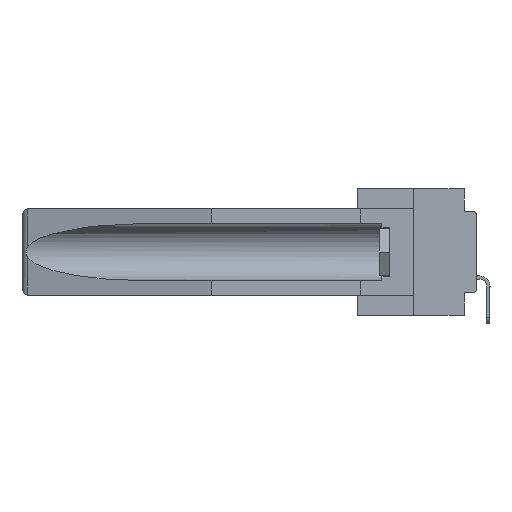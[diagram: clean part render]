
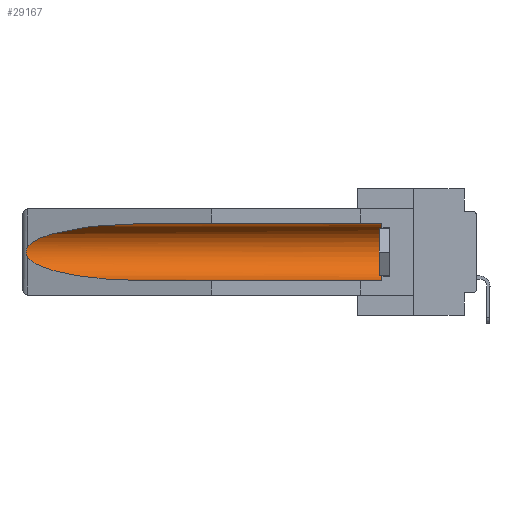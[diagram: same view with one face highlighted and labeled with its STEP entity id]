
A CAD part, left-side view. The second image highlights one B-rep face of the part: STEP entity #29167.
In plain terms, the highlighted cylindrical face has radius 2.857 mm (diameter 5.715 mm), a partial arc.
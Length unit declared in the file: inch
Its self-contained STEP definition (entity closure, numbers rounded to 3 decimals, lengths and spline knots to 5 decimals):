
#1202 = CARTESIAN_POINT ( 'NONE',  ( 0.26597, 1.5296, -0.19026 ) ) ;
#1560 = CARTESIAN_POINT ( 'NONE',  ( 0.21114, 1.30732, -0.284 ) ) ;
#1847 = AXIS2_PLACEMENT_3D ( 'NONE', #2452, #24636, #7703 ) ;
#2257 =( BOUNDED_CURVE ( )  B_SPLINE_CURVE ( 3, ( #26193, #17725, #25839, #3840 ),
 .UNSPECIFIED., .F., .F. ) 
 B_SPLINE_CURVE_WITH_KNOTS ( ( 4, 4 ),
 ( 4.71239, 6.08839 ),
 .UNSPECIFIED. ) 
 CURVE ( )  GEOMETRIC_REPRESENTATION_ITEM ( )  RATIONAL_B_SPLINE_CURVE ( ( 1., 0.848, 0.848, 1. ) ) 
 REPRESENTATION_ITEM ( '' )  );
#2452 = CARTESIAN_POINT ( 'NONE',  ( 0.155, -0.30754, -0.1715 ) ) ;
#2666 = EDGE_CURVE ( 'NONE', #32595, #31983, #2257, .T. ) ;
#3594 = VERTEX_POINT ( 'NONE', #14603 ) ;
#3840 = CARTESIAN_POINT ( 'NONE',  ( 0.26537, 1.52718, -0.14972 ) ) ;
#4075 = CIRCLE ( 'NONE', #16179, 0.1125 ) ;
#4083 = CARTESIAN_POINT ( 'NONE',  ( 0.26655, 1.53094, -0.18657 ) ) ;
#4867 = LINE ( 'NONE', #29758, #33152 ) ;
#6982 = EDGE_LOOP ( 'NONE', ( #12656, #14835, #35132, #25959, #32032, #20372 ) ) ;
#7193 = LINE ( 'NONE', #20549, #9250 ) ;
#7543 =( BOUNDED_CURVE ( )  B_SPLINE_CURVE ( 3, ( #23751, #20517, #1560, #31512 ),
 .UNSPECIFIED., .F., .F. ) 
 B_SPLINE_CURVE_WITH_KNOTS ( ( 4, 4 ),
 ( 0.1948, 1.5708 ),
 .UNSPECIFIED. ) 
 CURVE ( )  GEOMETRIC_REPRESENTATION_ITEM ( )  RATIONAL_B_SPLINE_CURVE ( ( 1., 0.848, 0.848, 1. ) ) 
 REPRESENTATION_ITEM ( '' )  );
#7703 = DIRECTION ( 'NONE',  ( 0., 0., 1. ) ) ;
#7984 = B_SPLINE_CURVE_WITH_KNOTS ( 'NONE', 3,
 ( #17441, #28968, #20332, #14750, #31323, #28789, #28255, #4083, #1202, #12393 ),
 .UNSPECIFIED., .F., .F.,
 ( 4, 2, 2, 2, 4 ),
 ( 0., 0.00029, 0.00058, 0.00087, 0.00117 ),
 .UNSPECIFIED. ) ;
#9250 = VECTOR ( 'NONE', #15162, 39.37008 ) ;
#10125 = CARTESIAN_POINT ( 'NONE',  ( 0.155, 0.126, -0.284 ) ) ;
#10772 = VERTEX_POINT ( 'NONE', #26915 ) ;
#11515 = EDGE_CURVE ( 'NONE', #10772, #3594, #7543, .T. ) ;
#12393 = CARTESIAN_POINT ( 'NONE',  ( 0.26537, 1.52718, -0.19328 ) ) ;
#12656 = ORIENTED_EDGE ( 'NONE', *, *, #2666, .T. ) ;
#14603 = CARTESIAN_POINT ( 'NONE',  ( 0.155, 1.07973, -0.284 ) ) ;
#14750 = CARTESIAN_POINT ( 'NONE',  ( 0.2673, 1.5327, -0.16383 ) ) ;
#14835 = ORIENTED_EDGE ( 'NONE', *, *, #24564, .T. ) ;
#15162 = DIRECTION ( 'NONE',  ( 0., 1., 0. ) ) ;
#16179 = AXIS2_PLACEMENT_3D ( 'NONE', #34949, #31898, #29348 ) ;
#16348 = EDGE_CURVE ( 'NONE', #18946, #3594, #4867, .T. ) ;
#16714 = FACE_OUTER_BOUND ( 'NONE', #6982, .T. ) ;
#17441 = CARTESIAN_POINT ( 'NONE',  ( 0.26537, 1.52718, -0.14972 ) ) ;
#17725 = CARTESIAN_POINT ( 'NONE',  ( 0.21114, 1.30732, -0.059 ) ) ;
#18946 = VERTEX_POINT ( 'NONE', #10125 ) ;
#20332 = CARTESIAN_POINT ( 'NONE',  ( 0.26654, 1.53092, -0.15636 ) ) ;
#20372 = ORIENTED_EDGE ( 'NONE', *, *, #20617, .T. ) ;
#20517 = CARTESIAN_POINT ( 'NONE',  ( 0.25451, 1.48313, -0.24835 ) ) ;
#20549 = CARTESIAN_POINT ( 'NONE',  ( 0.155, -0.30754, -0.059 ) ) ;
#20617 = EDGE_CURVE ( 'NONE', #28880, #32595, #7193, .T. ) ;
#22952 = EDGE_CURVE ( 'NONE', #18946, #28880, #4075, .T. ) ;
#23751 = CARTESIAN_POINT ( 'NONE',  ( 0.26537, 1.52718, -0.19328 ) ) ;
#24564 = EDGE_CURVE ( 'NONE', #31983, #10772, #7984, .T. ) ;
#24636 = DIRECTION ( 'NONE',  ( 0., 1., 0. ) ) ;
#24831 = CYLINDRICAL_SURFACE ( 'NONE', #1847, 0.1125 ) ;
#25839 = CARTESIAN_POINT ( 'NONE',  ( 0.25451, 1.48313, -0.09465 ) ) ;
#25959 = ORIENTED_EDGE ( 'NONE', *, *, #16348, .F. ) ;
#26193 = CARTESIAN_POINT ( 'NONE',  ( 0.155, 1.07973, -0.059 ) ) ;
#26869 = DIRECTION ( 'NONE',  ( 0., 1., 0. ) ) ;
#26915 = CARTESIAN_POINT ( 'NONE',  ( 0.26537, 1.52718, -0.19328 ) ) ;
#28255 = CARTESIAN_POINT ( 'NONE',  ( 0.2673, 1.53269, -0.17917 ) ) ;
#28539 = CARTESIAN_POINT ( 'NONE',  ( 0.155, 1.07973, -0.059 ) ) ;
#28627 = CARTESIAN_POINT ( 'NONE',  ( 0.155, 0.126, -0.059 ) ) ;
#28789 = CARTESIAN_POINT ( 'NONE',  ( 0.2675, 1.53308, -0.17534 ) ) ;
#28880 = VERTEX_POINT ( 'NONE', #28627 ) ;
#28968 = CARTESIAN_POINT ( 'NONE',  ( 0.26597, 1.52961, -0.15275 ) ) ;
#29167 = ADVANCED_FACE ( 'NONE', ( #16714 ), #24831, .F. ) ;
#29348 = DIRECTION ( 'NONE',  ( 0., 0., 1. ) ) ;
#29758 = CARTESIAN_POINT ( 'NONE',  ( 0.155, -0.30754, -0.284 ) ) ;
#31323 = CARTESIAN_POINT ( 'NONE',  ( 0.2675, 1.53308, -0.16763 ) ) ;
#31512 = CARTESIAN_POINT ( 'NONE',  ( 0.155, 1.07973, -0.284 ) ) ;
#31898 = DIRECTION ( 'NONE',  ( 0., -1., 0. ) ) ;
#31983 = VERTEX_POINT ( 'NONE', #33147 ) ;
#32032 = ORIENTED_EDGE ( 'NONE', *, *, #22952, .T. ) ;
#32595 = VERTEX_POINT ( 'NONE', #28539 ) ;
#33147 = CARTESIAN_POINT ( 'NONE',  ( 0.26537, 1.52718, -0.14972 ) ) ;
#33152 = VECTOR ( 'NONE', #26869, 39.37008 ) ;
#34949 = CARTESIAN_POINT ( 'NONE',  ( 0.155, 0.126, -0.1715 ) ) ;
#35132 = ORIENTED_EDGE ( 'NONE', *, *, #11515, .T. ) ;
